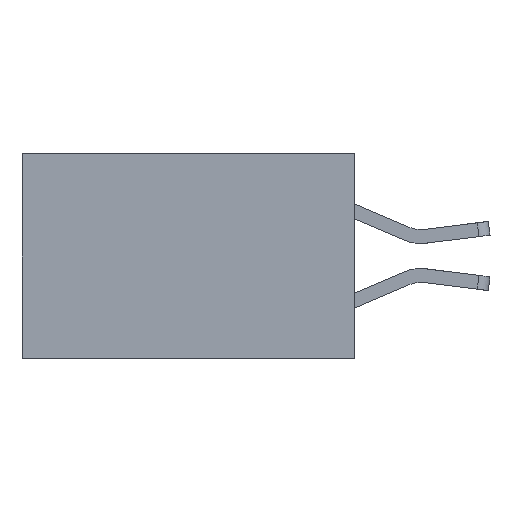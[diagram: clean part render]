
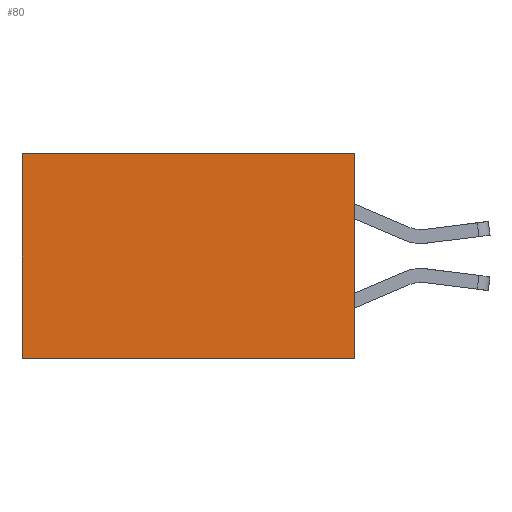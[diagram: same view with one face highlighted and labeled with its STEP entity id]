
A CAD part, left-side view. The second image highlights one B-rep face of the part: STEP entity #80.
In plain terms, the highlighted planar face has unit normal (-1, 0, 0).
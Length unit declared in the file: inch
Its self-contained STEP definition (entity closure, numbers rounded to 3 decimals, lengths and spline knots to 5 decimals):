
#80 = ADVANCED_FACE ( 'NONE', ( #4304 ), #1208, .F. ) ;
#139 = LINE ( 'NONE', #961, #3403 ) ;
#485 = DIRECTION ( 'NONE',  ( 1., 0., 0. ) ) ;
#521 = VERTEX_POINT ( 'NONE', #1249 ) ;
#751 = VERTEX_POINT ( 'NONE', #6367 ) ;
#828 = LINE ( 'NONE', #3195, #5580 ) ;
#961 = CARTESIAN_POINT ( 'NONE',  ( 0.2615, 0., -0.37 ) ) ;
#1028 = LINE ( 'NONE', #7226, #9986 ) ;
#1208 = PLANE ( 'NONE',  #5717 ) ;
#1249 = CARTESIAN_POINT ( 'NONE',  ( 0.2615, 0.6, -0.37 ) ) ;
#1369 = DIRECTION ( 'NONE',  ( 0., 0., -1. ) ) ;
#1991 = EDGE_CURVE ( 'NONE', #5227, #5786, #828, .T. ) ;
#2084 = EDGE_CURVE ( 'NONE', #5786, #521, #1028, .T. ) ;
#2439 = ORIENTED_EDGE ( 'NONE', *, *, #2084, .T. ) ;
#3040 = ORIENTED_EDGE ( 'NONE', *, *, #4292, .F. ) ;
#3195 = CARTESIAN_POINT ( 'NONE',  ( 0.2615, 0., 0. ) ) ;
#3221 = ORIENTED_EDGE ( 'NONE', *, *, #4536, .F. ) ;
#3403 = VECTOR ( 'NONE', #4262, 39.37008 ) ;
#3641 = CARTESIAN_POINT ( 'NONE',  ( 0.2615, 0., -0.37 ) ) ;
#3693 = CARTESIAN_POINT ( 'NONE',  ( 0.2615, 0.6, 0. ) ) ;
#4224 = VECTOR ( 'NONE', #7459, 39.37008 ) ;
#4262 = DIRECTION ( 'NONE',  ( 0., 1., 0. ) ) ;
#4292 = EDGE_CURVE ( 'NONE', #751, #521, #139, .T. ) ;
#4304 = FACE_OUTER_BOUND ( 'NONE', #5966, .T. ) ;
#4536 = EDGE_CURVE ( 'NONE', #5227, #751, #7629, .T. ) ;
#5227 = VERTEX_POINT ( 'NONE', #5909 ) ;
#5580 = VECTOR ( 'NONE', #6322, 39.37008 ) ;
#5636 = ORIENTED_EDGE ( 'NONE', *, *, #1991, .T. ) ;
#5658 = DIRECTION ( 'NONE',  ( 0., 0., -1. ) ) ;
#5717 = AXIS2_PLACEMENT_3D ( 'NONE', #8265, #485, #1369 ) ;
#5786 = VERTEX_POINT ( 'NONE', #3693 ) ;
#5909 = CARTESIAN_POINT ( 'NONE',  ( 0.2615, 0., 0. ) ) ;
#5966 = EDGE_LOOP ( 'NONE', ( #2439, #3040, #3221, #5636 ) ) ;
#6322 = DIRECTION ( 'NONE',  ( 0., 1., 0. ) ) ;
#6367 = CARTESIAN_POINT ( 'NONE',  ( 0.2615, 0., -0.37 ) ) ;
#7226 = CARTESIAN_POINT ( 'NONE',  ( 0.2615, 0.6, -0.37 ) ) ;
#7459 = DIRECTION ( 'NONE',  ( 0., 0., -1. ) ) ;
#7629 = LINE ( 'NONE', #3641, #4224 ) ;
#8265 = CARTESIAN_POINT ( 'NONE',  ( 0.2615, 0., -0.37 ) ) ;
#9986 = VECTOR ( 'NONE', #5658, 39.37008 ) ;
